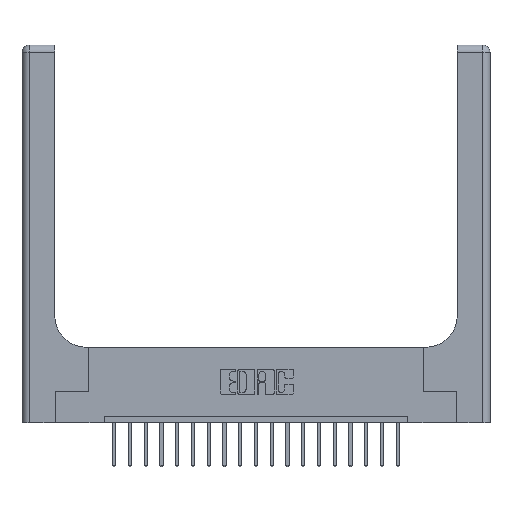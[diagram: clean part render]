
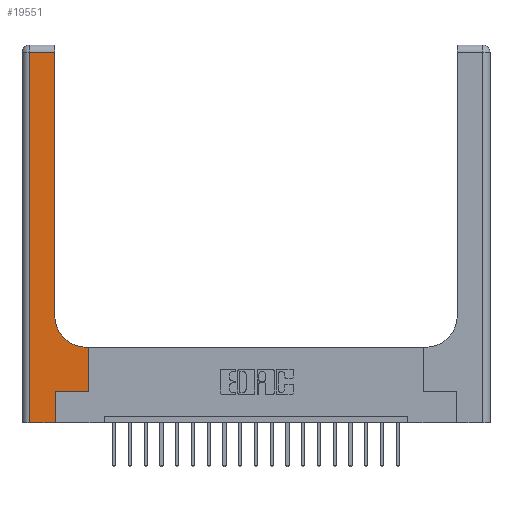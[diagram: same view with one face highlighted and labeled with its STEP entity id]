
A CAD part, top view. The second image highlights one B-rep face of the part: STEP entity #19551.
In plain terms, the highlighted planar face has unit normal (0, 0, 1).
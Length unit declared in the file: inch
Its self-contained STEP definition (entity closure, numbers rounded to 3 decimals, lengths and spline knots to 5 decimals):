
#166 = EDGE_CURVE ( 'NONE', #5883, #1383, #15339, .T. ) ;
#444 = DIRECTION ( 'NONE',  ( 0., 0., -1. ) ) ;
#671 = CARTESIAN_POINT ( 'NONE',  ( 0., 2.94, 0.37 ) ) ;
#997 = CARTESIAN_POINT ( 'NONE',  ( 0.528, 0.6, 0.37 ) ) ;
#1175 = DIRECTION ( 'NONE',  ( -1., 0., 0. ) ) ;
#1331 = VECTOR ( 'NONE', #6145, 39.37008 ) ;
#1383 = VERTEX_POINT ( 'NONE', #997 ) ;
#2191 = EDGE_LOOP ( 'NONE', ( #17872, #18368, #5458, #16152, #15823, #14709, #12995, #4182, #7515 ) ) ;
#2358 = EDGE_CURVE ( 'NONE', #13009, #19728, #10679, .T. ) ;
#2400 = CARTESIAN_POINT ( 'NONE',  ( 0.06, 0., 0.37 ) ) ;
#2745 = DIRECTION ( 'NONE',  ( 0., 0., -1. ) ) ;
#2755 = CARTESIAN_POINT ( 'NONE',  ( 0.26, 0.6, 0.37 ) ) ;
#2762 = CARTESIAN_POINT ( 'NONE',  ( 0.06, 3., 0.37 ) ) ;
#3315 = CARTESIAN_POINT ( 'NONE',  ( 0.528, 0.25, 0.37 ) ) ;
#3323 = CARTESIAN_POINT ( 'NONE',  ( 0.06, 2.94, 0.37 ) ) ;
#3936 = EDGE_CURVE ( 'NONE', #19393, #12786, #6495, .T. ) ;
#4168 = DIRECTION ( 'NONE',  ( 1., 0., 0. ) ) ;
#4182 = ORIENTED_EDGE ( 'NONE', *, *, #14434, .T. ) ;
#4490 = EDGE_CURVE ( 'NONE', #5861, #19393, #14246, .T. ) ;
#4580 = VECTOR ( 'NONE', #19950, 39.37008 ) ;
#5092 = PLANE ( 'NONE',  #14997 ) ;
#5290 = CARTESIAN_POINT ( 'NONE',  ( 0.265, 0.25, 0.37 ) ) ;
#5458 = ORIENTED_EDGE ( 'NONE', *, *, #3936, .T. ) ;
#5861 = VERTEX_POINT ( 'NONE', #6584 ) ;
#5883 = VERTEX_POINT ( 'NONE', #12939 ) ;
#6145 = DIRECTION ( 'NONE',  ( 1., 0., 0. ) ) ;
#6495 = LINE ( 'NONE', #2762, #4580 ) ;
#6584 = CARTESIAN_POINT ( 'NONE',  ( 0.26, 2.94, 0.37 ) ) ;
#6813 = FACE_OUTER_BOUND ( 'NONE', #2191, .T. ) ;
#7348 = VECTOR ( 'NONE', #15678, 39.37008 ) ;
#7360 = EDGE_CURVE ( 'NONE', #19728, #5861, #17523, .T. ) ;
#7515 = ORIENTED_EDGE ( 'NONE', *, *, #2358, .T. ) ;
#7932 = EDGE_CURVE ( 'NONE', #12786, #14496, #18226, .T. ) ;
#8047 = VECTOR ( 'NONE', #4168, 39.37008 ) ;
#8164 = EDGE_CURVE ( 'NONE', #14496, #17934, #15772, .T. ) ;
#8806 = CARTESIAN_POINT ( 'NONE',  ( 0., 0., 0.37 ) ) ;
#8810 = DIRECTION ( 'NONE',  ( 1., 0., 0. ) ) ;
#9218 = DIRECTION ( 'NONE',  ( 0., 1., 0. ) ) ;
#9285 = CARTESIAN_POINT ( 'NONE',  ( 0.26, 3., 0.37 ) ) ;
#10679 = CIRCLE ( 'NONE', #12315, 0.25 ) ;
#10807 = CARTESIAN_POINT ( 'NONE',  ( 0.265, 0.25, 0.37 ) ) ;
#11290 = DIRECTION ( 'NONE',  ( -1., 0., 0. ) ) ;
#12315 = AXIS2_PLACEMENT_3D ( 'NONE', #19584, #2745, #8810 ) ;
#12786 = VERTEX_POINT ( 'NONE', #2400 ) ;
#12939 = CARTESIAN_POINT ( 'NONE',  ( 0.528, 0.25, 0.37 ) ) ;
#12995 = ORIENTED_EDGE ( 'NONE', *, *, #166, .T. ) ;
#13009 = VERTEX_POINT ( 'NONE', #13865 ) ;
#13370 = VECTOR ( 'NONE', #9218, 39.37008 ) ;
#13865 = CARTESIAN_POINT ( 'NONE',  ( 0.51, 0.6, 0.37 ) ) ;
#14246 = LINE ( 'NONE', #671, #20080 ) ;
#14434 = EDGE_CURVE ( 'NONE', #1383, #13009, #17682, .T. ) ;
#14496 = VERTEX_POINT ( 'NONE', #18388 ) ;
#14709 = ORIENTED_EDGE ( 'NONE', *, *, #18250, .T. ) ;
#14773 = VECTOR ( 'NONE', #1175, 39.37008 ) ;
#14997 = AXIS2_PLACEMENT_3D ( 'NONE', #15877, #444, #11290 ) ;
#15339 = LINE ( 'NONE', #3315, #7348 ) ;
#15678 = DIRECTION ( 'NONE',  ( 0., 1., 0. ) ) ;
#15706 = DIRECTION ( 'NONE',  ( 0., 1., 0. ) ) ;
#15772 = LINE ( 'NONE', #15775, #18449 ) ;
#15775 = CARTESIAN_POINT ( 'NONE',  ( 0.265, 0., 0.37 ) ) ;
#15823 = ORIENTED_EDGE ( 'NONE', *, *, #8164, .T. ) ;
#15877 = CARTESIAN_POINT ( 'NONE',  ( 0., 3., 0.37 ) ) ;
#16152 = ORIENTED_EDGE ( 'NONE', *, *, #7932, .T. ) ;
#16175 = DIRECTION ( 'NONE',  ( -1., 0., 0. ) ) ;
#17523 = LINE ( 'NONE', #9285, #13370 ) ;
#17682 = LINE ( 'NONE', #2755, #14773 ) ;
#17795 = LINE ( 'NONE', #10807, #1331 ) ;
#17872 = ORIENTED_EDGE ( 'NONE', *, *, #7360, .T. ) ;
#17934 = VERTEX_POINT ( 'NONE', #5290 ) ;
#18098 = CARTESIAN_POINT ( 'NONE',  ( 0.26, 0.85, 0.37 ) ) ;
#18226 = LINE ( 'NONE', #8806, #8047 ) ;
#18250 = EDGE_CURVE ( 'NONE', #17934, #5883, #17795, .T. ) ;
#18368 = ORIENTED_EDGE ( 'NONE', *, *, #4490, .T. ) ;
#18388 = CARTESIAN_POINT ( 'NONE',  ( 0.265, 0., 0.37 ) ) ;
#18449 = VECTOR ( 'NONE', #15706, 39.37008 ) ;
#19393 = VERTEX_POINT ( 'NONE', #3323 ) ;
#19551 = ADVANCED_FACE ( 'NONE', ( #6813 ), #5092, .F. ) ;
#19584 = CARTESIAN_POINT ( 'NONE',  ( 0.51, 0.85, 0.37 ) ) ;
#19728 = VERTEX_POINT ( 'NONE', #18098 ) ;
#19950 = DIRECTION ( 'NONE',  ( 0., -1., 0. ) ) ;
#20080 = VECTOR ( 'NONE', #16175, 39.37008 ) ;
